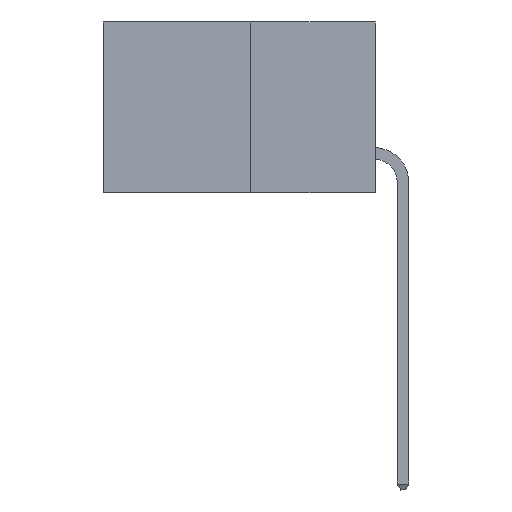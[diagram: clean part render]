
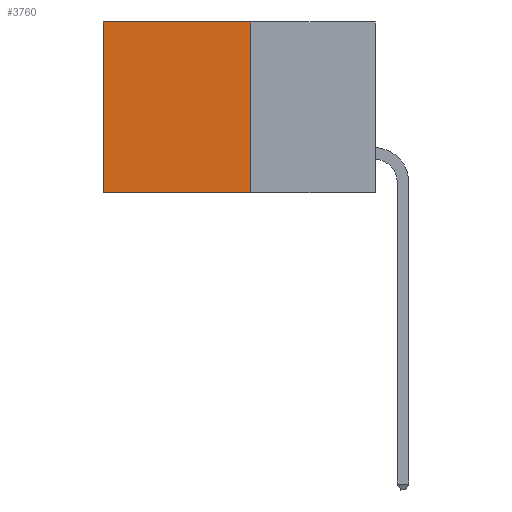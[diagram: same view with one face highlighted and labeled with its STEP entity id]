
A CAD part, left-side view. The second image highlights one B-rep face of the part: STEP entity #3760.
In plain terms, the highlighted planar face has unit normal (-1, 0, 0).
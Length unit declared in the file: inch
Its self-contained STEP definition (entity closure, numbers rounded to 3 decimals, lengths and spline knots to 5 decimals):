
#289 = VERTEX_POINT ( 'NONE', #6617 ) ;
#727 = CARTESIAN_POINT ( 'NONE',  ( 0.277, 0.27, 0. ) ) ;
#1908 = VECTOR ( 'NONE', #3396, 39.37008 ) ;
#1973 = VERTEX_POINT ( 'NONE', #9725 ) ;
#2546 = EDGE_CURVE ( 'NONE', #1973, #289, #12778, .T. ) ;
#2803 = EDGE_CURVE ( 'NONE', #6841, #289, #8044, .T. ) ;
#3396 = DIRECTION ( 'NONE',  ( 0., 0., -1. ) ) ;
#3570 = VECTOR ( 'NONE', #7314, 39.37008 ) ;
#3607 = EDGE_CURVE ( 'NONE', #11488, #1973, #12353, .T. ) ;
#3760 = ADVANCED_FACE ( 'NONE', ( #10950 ), #9622, .F. ) ;
#5248 = AXIS2_PLACEMENT_3D ( 'NONE', #9447, #9303, #9429 ) ;
#5926 = VECTOR ( 'NONE', #14978, 39.37008 ) ;
#6617 = CARTESIAN_POINT ( 'NONE',  ( 0.277, 0.59, -0.37 ) ) ;
#6841 = VERTEX_POINT ( 'NONE', #7204 ) ;
#7204 = CARTESIAN_POINT ( 'NONE',  ( 0.277, 0.27, -0.37 ) ) ;
#7314 = DIRECTION ( 'NONE',  ( 0., 0., -1. ) ) ;
#7644 = VECTOR ( 'NONE', #10951, 39.37008 ) ;
#8004 = ORIENTED_EDGE ( 'NONE', *, *, #2546, .T. ) ;
#8044 = LINE ( 'NONE', #11230, #7644 ) ;
#8439 = ORIENTED_EDGE ( 'NONE', *, *, #2803, .F. ) ;
#8708 = LINE ( 'NONE', #9312, #1908 ) ;
#9303 = DIRECTION ( 'NONE',  ( 1., 0., 0. ) ) ;
#9312 = CARTESIAN_POINT ( 'NONE',  ( 0.277, 0.27, -0.37 ) ) ;
#9409 = ORIENTED_EDGE ( 'NONE', *, *, #10948, .F. ) ;
#9429 = DIRECTION ( 'NONE',  ( 0., 0., -1. ) ) ;
#9447 = CARTESIAN_POINT ( 'NONE',  ( 0.277, 0.27, -0.37 ) ) ;
#9622 = PLANE ( 'NONE',  #5248 ) ;
#9646 = ORIENTED_EDGE ( 'NONE', *, *, #3607, .T. ) ;
#9662 = CARTESIAN_POINT ( 'NONE',  ( 0.277, 0.59, -0.37 ) ) ;
#9725 = CARTESIAN_POINT ( 'NONE',  ( 0.277, 0.59, 0. ) ) ;
#10045 = EDGE_LOOP ( 'NONE', ( #8004, #8439, #9409, #9646 ) ) ;
#10948 = EDGE_CURVE ( 'NONE', #11488, #6841, #8708, .T. ) ;
#10950 = FACE_OUTER_BOUND ( 'NONE', #10045, .T. ) ;
#10951 = DIRECTION ( 'NONE',  ( 0., 1., 0. ) ) ;
#11230 = CARTESIAN_POINT ( 'NONE',  ( 0.277, 0.27, -0.37 ) ) ;
#11488 = VERTEX_POINT ( 'NONE', #727 ) ;
#12353 = LINE ( 'NONE', #15117, #5926 ) ;
#12778 = LINE ( 'NONE', #9662, #3570 ) ;
#14978 = DIRECTION ( 'NONE',  ( 0., 1., 0. ) ) ;
#15117 = CARTESIAN_POINT ( 'NONE',  ( 0.277, 0.27, 0. ) ) ;
